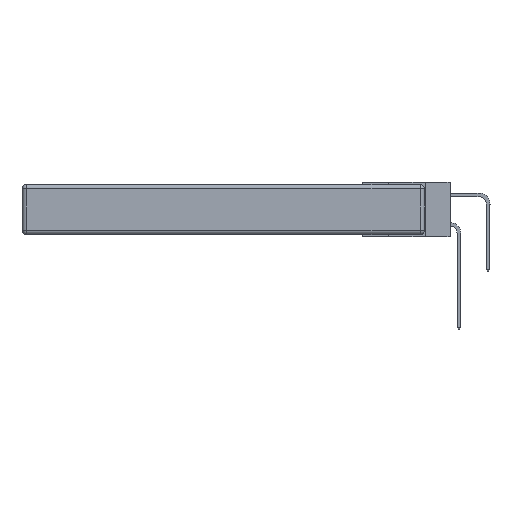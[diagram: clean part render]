
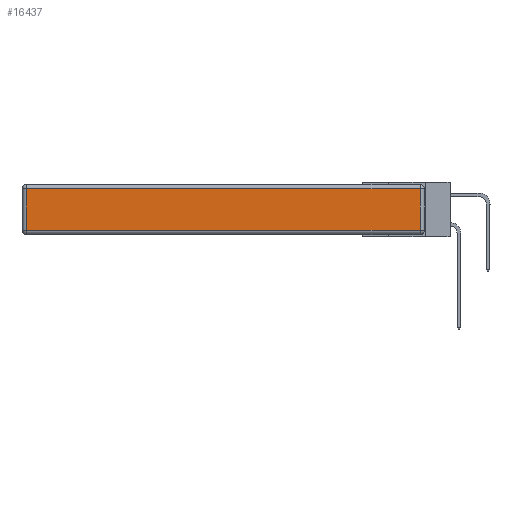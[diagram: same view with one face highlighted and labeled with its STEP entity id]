
A CAD part, left-side view. The second image highlights one B-rep face of the part: STEP entity #16437.
In plain terms, the highlighted planar face has unit normal (-1, 0, 0).
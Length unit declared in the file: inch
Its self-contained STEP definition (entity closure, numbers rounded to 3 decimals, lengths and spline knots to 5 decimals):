
#138 = VERTEX_POINT ( 'NONE', #11675 ) ;
#715 = EDGE_CURVE ( 'NONE', #13929, #15900, #8401, .T. ) ;
#1423 = LINE ( 'NONE', #15489, #15789 ) ;
#1511 = DIRECTION ( 'NONE',  ( 0., 0., 1. ) ) ;
#1532 = EDGE_LOOP ( 'NONE', ( #17347, #7871, #2597, #12110 ) ) ;
#1771 = CARTESIAN_POINT ( 'NONE',  ( 0., 0.03, -0.343 ) ) ;
#2222 = DIRECTION ( 'NONE',  ( 0., -1., 0. ) ) ;
#2597 = ORIENTED_EDGE ( 'NONE', *, *, #9043, .T. ) ;
#2673 = CARTESIAN_POINT ( 'NONE',  ( 0., 2.72, -0.313 ) ) ;
#5230 = CARTESIAN_POINT ( 'NONE',  ( 0., 2.72, -0.343 ) ) ;
#5512 = LINE ( 'NONE', #17670, #7102 ) ;
#7102 = VECTOR ( 'NONE', #16327, 39.37008 ) ;
#7871 = ORIENTED_EDGE ( 'NONE', *, *, #715, .T. ) ;
#8401 = LINE ( 'NONE', #1771, #14019 ) ;
#9043 = EDGE_CURVE ( 'NONE', #15900, #138, #5512, .T. ) ;
#9537 = EDGE_CURVE ( 'NONE', #138, #13506, #16783, .T. ) ;
#9864 = DIRECTION ( 'NONE',  ( 0., 0., -1. ) ) ;
#11675 = CARTESIAN_POINT ( 'NONE',  ( 0., 2.72, -0.03 ) ) ;
#11801 = DIRECTION ( 'NONE',  ( -1., 0., 0. ) ) ;
#12110 = ORIENTED_EDGE ( 'NONE', *, *, #9537, .T. ) ;
#13506 = VERTEX_POINT ( 'NONE', #2673 ) ;
#13913 = FACE_OUTER_BOUND ( 'NONE', #1532, .T. ) ;
#13929 = VERTEX_POINT ( 'NONE', #16877 ) ;
#14019 = VECTOR ( 'NONE', #1511, 39.37008 ) ;
#14977 = EDGE_CURVE ( 'NONE', #13506, #13929, #1423, .T. ) ;
#15489 = CARTESIAN_POINT ( 'NONE',  ( 0., 0., -0.313 ) ) ;
#15789 = VECTOR ( 'NONE', #2222, 39.37008 ) ;
#15900 = VERTEX_POINT ( 'NONE', #19110 ) ;
#16124 = PLANE ( 'NONE',  #16794 ) ;
#16327 = DIRECTION ( 'NONE',  ( 0., 1., 0. ) ) ;
#16437 = ADVANCED_FACE ( 'NONE', ( #13913 ), #16124, .T. ) ;
#16783 = LINE ( 'NONE', #5230, #19094 ) ;
#16794 = AXIS2_PLACEMENT_3D ( 'NONE', #17573, #11801, #19085 ) ;
#16877 = CARTESIAN_POINT ( 'NONE',  ( 0., 0.03, -0.313 ) ) ;
#17347 = ORIENTED_EDGE ( 'NONE', *, *, #14977, .T. ) ;
#17573 = CARTESIAN_POINT ( 'NONE',  ( 0., 0., -0.343 ) ) ;
#17670 = CARTESIAN_POINT ( 'NONE',  ( 0., 2.75, -0.03 ) ) ;
#19085 = DIRECTION ( 'NONE',  ( 0., 0., 1. ) ) ;
#19094 = VECTOR ( 'NONE', #9864, 39.37008 ) ;
#19110 = CARTESIAN_POINT ( 'NONE',  ( 0., 0.03, -0.03 ) ) ;
